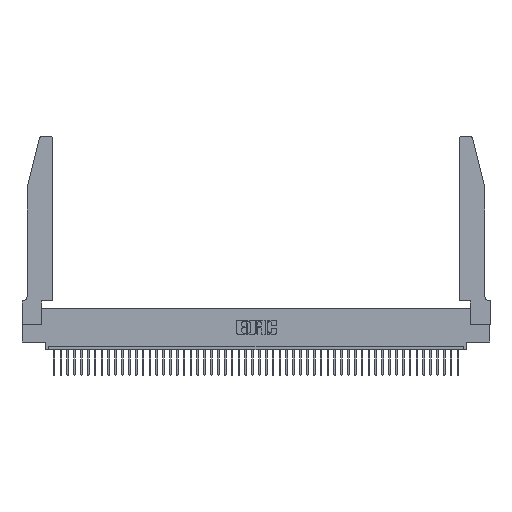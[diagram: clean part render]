
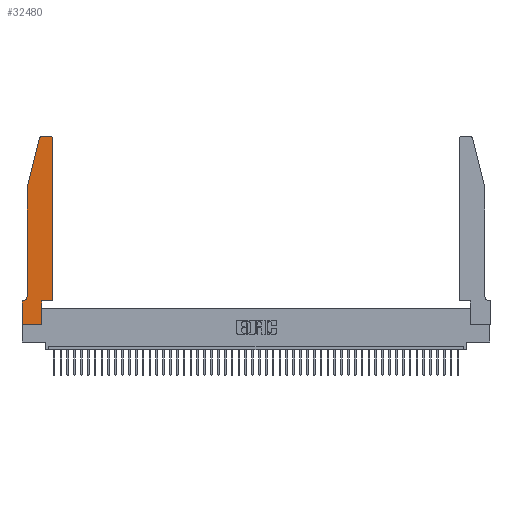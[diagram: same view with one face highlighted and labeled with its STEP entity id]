
A CAD part, top view. The second image highlights one B-rep face of the part: STEP entity #32480.
In plain terms, the highlighted planar face has unit normal (0, 0, 1).
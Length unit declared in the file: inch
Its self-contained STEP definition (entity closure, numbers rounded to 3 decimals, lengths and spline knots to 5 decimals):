
#525 = ORIENTED_EDGE ( 'NONE', *, *, #40745, .T. ) ;
#1205 = ORIENTED_EDGE ( 'NONE', *, *, #20971, .T. ) ;
#1322 = ORIENTED_EDGE ( 'NONE', *, *, #21692, .T. ) ;
#2195 = DIRECTION ( 'NONE',  ( -0.239, -0.971, 0. ) ) ;
#2230 = ORIENTED_EDGE ( 'NONE', *, *, #13888, .T. ) ;
#2382 = DIRECTION ( 'NONE',  ( 1., 0., 0. ) ) ;
#2586 = VERTEX_POINT ( 'NONE', #12511 ) ;
#2646 = VERTEX_POINT ( 'NONE', #35021 ) ;
#2948 = VECTOR ( 'NONE', #14904, 39.37008 ) ;
#3044 = AXIS2_PLACEMENT_3D ( 'NONE', #18014, #7281, #39890 ) ;
#4023 = CARTESIAN_POINT ( 'NONE',  ( 0.0755, 0.35, 0.37 ) ) ;
#4168 = CARTESIAN_POINT ( 'NONE',  ( 0., 0., 0.37 ) ) ;
#4309 = DIRECTION ( 'NONE',  ( 1., 0., 0. ) ) ;
#4430 = ORIENTED_EDGE ( 'NONE', *, *, #29819, .T. ) ;
#4455 = FACE_OUTER_BOUND ( 'NONE', #10011, .T. ) ;
#4834 = LINE ( 'NONE', #19809, #19164 ) ;
#5432 = EDGE_CURVE ( 'NONE', #11202, #2646, #16679, .T. ) ;
#5494 = VECTOR ( 'NONE', #2195, 39.37008 ) ;
#5593 = CARTESIAN_POINT ( 'NONE',  ( 0.2865, 0.35, 0.37 ) ) ;
#5926 = DIRECTION ( 'NONE',  ( 0., 0., 1. ) ) ;
#6173 = ORIENTED_EDGE ( 'NONE', *, *, #10492, .T. ) ;
#6420 = DIRECTION ( 'NONE',  ( 1., 0., 0. ) ) ;
#7226 = VECTOR ( 'NONE', #20604, 39.37008 ) ;
#7281 = DIRECTION ( 'NONE',  ( 0., 0., -1. ) ) ;
#8592 = DIRECTION ( 'NONE',  ( 0., 1., 0. ) ) ;
#9051 = CARTESIAN_POINT ( 'NONE',  ( 0.0755, 2., 0.37 ) ) ;
#9161 = EDGE_CURVE ( 'NONE', #2586, #29122, #30845, .T. ) ;
#9320 = CIRCLE ( 'NONE', #40658, 0.03 ) ;
#9470 = VERTEX_POINT ( 'NONE', #18917 ) ;
#10011 = EDGE_LOOP ( 'NONE', ( #6173, #20983, #21105, #4430, #1322, #1205, #36152, #15842, #525, #2230, #44123, #16639 ) ) ;
#10123 = DIRECTION ( 'NONE',  ( 1., 0., 0. ) ) ;
#10492 = EDGE_CURVE ( 'NONE', #18488, #15347, #18640, .T. ) ;
#10690 = VERTEX_POINT ( 'NONE', #11948 ) ;
#10812 = EDGE_CURVE ( 'NONE', #10690, #46257, #42287, .T. ) ;
#11202 = VERTEX_POINT ( 'NONE', #23152 ) ;
#11948 = CARTESIAN_POINT ( 'NONE',  ( 0.25487, 2.72718, 0.37 ) ) ;
#12471 = EDGE_CURVE ( 'NONE', #15347, #10690, #9320, .T. ) ;
#12511 = CARTESIAN_POINT ( 'NONE',  ( 0.4505, 0.35, 0.37 ) ) ;
#12670 = LINE ( 'NONE', #40149, #2948 ) ;
#13855 = CIRCLE ( 'NONE', #21429, 0.03 ) ;
#13888 = EDGE_CURVE ( 'NONE', #45760, #2586, #44239, .T. ) ;
#14904 = DIRECTION ( 'NONE',  ( 0., -1., 0. ) ) ;
#15347 = VERTEX_POINT ( 'NONE', #33865 ) ;
#15842 = ORIENTED_EDGE ( 'NONE', *, *, #5432, .T. ) ;
#16373 = VECTOR ( 'NONE', #21807, 39.37008 ) ;
#16639 = ORIENTED_EDGE ( 'NONE', *, *, #42697, .T. ) ;
#16679 = LINE ( 'NONE', #24708, #27622 ) ;
#16923 = CARTESIAN_POINT ( 'NONE',  ( 0.2605, 2.75, 0.37 ) ) ;
#18014 = CARTESIAN_POINT ( 'NONE',  ( 0.0055, 0.42, 0.37 ) ) ;
#18488 = VERTEX_POINT ( 'NONE', #40890 ) ;
#18640 = LINE ( 'NONE', #16923, #7226 ) ;
#18917 = CARTESIAN_POINT ( 'NONE',  ( 0.0755, 0.42, 0.37 ) ) ;
#19042 = DIRECTION ( 'NONE',  ( 0., 0., 1. ) ) ;
#19164 = VECTOR ( 'NONE', #41865, 39.37008 ) ;
#19809 = CARTESIAN_POINT ( 'NONE',  ( 0.2865, 0.35, 0.37 ) ) ;
#20279 = CARTESIAN_POINT ( 'NONE',  ( 0., 0.35, 0.37 ) ) ;
#20473 = CARTESIAN_POINT ( 'NONE',  ( 0.0755, 2., 0.37 ) ) ;
#20604 = DIRECTION ( 'NONE',  ( -1., 0., 0. ) ) ;
#20971 = EDGE_CURVE ( 'NONE', #22901, #23405, #27310, .T. ) ;
#20983 = ORIENTED_EDGE ( 'NONE', *, *, #12471, .T. ) ;
#21105 = ORIENTED_EDGE ( 'NONE', *, *, #10812, .T. ) ;
#21429 = AXIS2_PLACEMENT_3D ( 'NONE', #33867, #19042, #34034 ) ;
#21692 = EDGE_CURVE ( 'NONE', #9470, #22901, #30311, .T. ) ;
#21807 = DIRECTION ( 'NONE',  ( -1., 0., 0. ) ) ;
#22901 = VERTEX_POINT ( 'NONE', #37897 ) ;
#23152 = CARTESIAN_POINT ( 'NONE',  ( 0., 0., 0.37 ) ) ;
#23405 = VERTEX_POINT ( 'NONE', #20279 ) ;
#23504 = CARTESIAN_POINT ( 'NONE',  ( 0.4505, 0.35, 0.37 ) ) ;
#24708 = CARTESIAN_POINT ( 'NONE',  ( 0., 0., 0.37 ) ) ;
#25979 = PLANE ( 'NONE',  #31687 ) ;
#26214 = VECTOR ( 'NONE', #8592, 39.37008 ) ;
#27310 = LINE ( 'NONE', #4023, #16373 ) ;
#27622 = VECTOR ( 'NONE', #6420, 39.37008 ) ;
#29122 = VERTEX_POINT ( 'NONE', #38073 ) ;
#29819 = EDGE_CURVE ( 'NONE', #46257, #9470, #12670, .T. ) ;
#29939 = VECTOR ( 'NONE', #40619, 39.37008 ) ;
#30311 = CIRCLE ( 'NONE', #3044, 0.07 ) ;
#30845 = LINE ( 'NONE', #23504, #26214 ) ;
#31687 = AXIS2_PLACEMENT_3D ( 'NONE', #37069, #33840, #4309 ) ;
#32480 = ADVANCED_FACE ( 'NONE', ( #4455 ), #25979, .T. ) ;
#33840 = DIRECTION ( 'NONE',  ( 0., 0., 1. ) ) ;
#33865 = CARTESIAN_POINT ( 'NONE',  ( 0.284, 2.75, 0.37 ) ) ;
#33867 = CARTESIAN_POINT ( 'NONE',  ( 0.4205, 2.72, 0.37 ) ) ;
#33957 = LINE ( 'NONE', #4168, #29939 ) ;
#34034 = DIRECTION ( 'NONE',  ( 1., 0., 0. ) ) ;
#35021 = CARTESIAN_POINT ( 'NONE',  ( 0.2865, 0., 0.37 ) ) ;
#36152 = ORIENTED_EDGE ( 'NONE', *, *, #39936, .T. ) ;
#37069 = CARTESIAN_POINT ( 'NONE',  ( 0., 0.35, 0.37 ) ) ;
#37897 = CARTESIAN_POINT ( 'NONE',  ( 0.0055, 0.35, 0.37 ) ) ;
#38073 = CARTESIAN_POINT ( 'NONE',  ( 0.4505, 2.72, 0.37 ) ) ;
#39161 = CARTESIAN_POINT ( 'NONE',  ( 0.284, 2.72, 0.37 ) ) ;
#39890 = DIRECTION ( 'NONE',  ( -1., 0., 0. ) ) ;
#39936 = EDGE_CURVE ( 'NONE', #23405, #11202, #33957, .T. ) ;
#40149 = CARTESIAN_POINT ( 'NONE',  ( 0.0755, 2., 0.37 ) ) ;
#40619 = DIRECTION ( 'NONE',  ( 0., -1., 0. ) ) ;
#40658 = AXIS2_PLACEMENT_3D ( 'NONE', #39161, #5926, #2382 ) ;
#40745 = EDGE_CURVE ( 'NONE', #2646, #45760, #4834, .T. ) ;
#40772 = VECTOR ( 'NONE', #10123, 39.37008 ) ;
#40890 = CARTESIAN_POINT ( 'NONE',  ( 0.4205, 2.75, 0.37 ) ) ;
#41865 = DIRECTION ( 'NONE',  ( 0., 1., 0. ) ) ;
#42287 = LINE ( 'NONE', #20473, #5494 ) ;
#42697 = EDGE_CURVE ( 'NONE', #29122, #18488, #13855, .T. ) ;
#44123 = ORIENTED_EDGE ( 'NONE', *, *, #9161, .T. ) ;
#44239 = LINE ( 'NONE', #45840, #40772 ) ;
#45760 = VERTEX_POINT ( 'NONE', #5593 ) ;
#45840 = CARTESIAN_POINT ( 'NONE',  ( 0.4505, 0.35, 0.37 ) ) ;
#46257 = VERTEX_POINT ( 'NONE', #9051 ) ;
